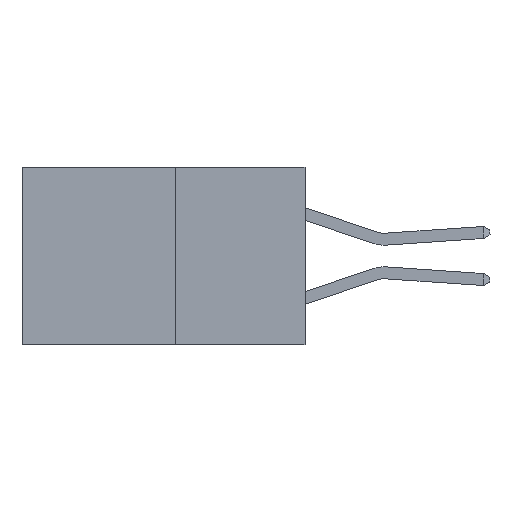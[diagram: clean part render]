
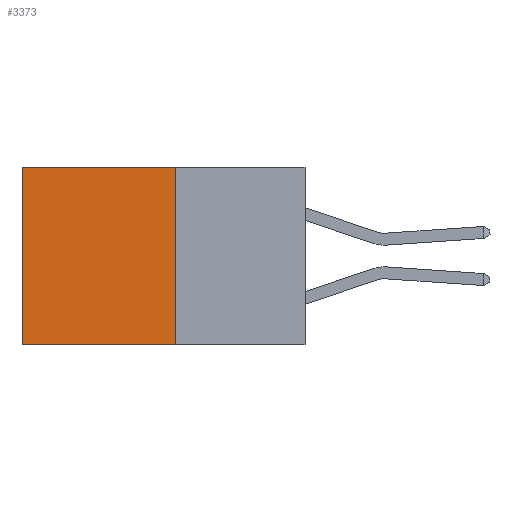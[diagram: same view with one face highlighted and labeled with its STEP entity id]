
A CAD part, left-side view. The second image highlights one B-rep face of the part: STEP entity #3373.
In plain terms, the highlighted planar face has unit normal (-1, 0, 0).
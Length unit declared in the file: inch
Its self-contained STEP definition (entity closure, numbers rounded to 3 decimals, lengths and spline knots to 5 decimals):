
#1006 = CARTESIAN_POINT ( 'NONE',  ( 0.277, 0.59, 0. ) ) ;
#1196 = CARTESIAN_POINT ( 'NONE',  ( 0.277, 0.59, -0.37 ) ) ;
#2327 = EDGE_CURVE ( 'NONE', #13616, #3309, #2424, .T. ) ;
#2424 = LINE ( 'NONE', #1196, #14204 ) ;
#3309 = VERTEX_POINT ( 'NONE', #13774 ) ;
#3373 = ADVANCED_FACE ( 'NONE', ( #16665 ), #11764, .F. ) ;
#3637 = VECTOR ( 'NONE', #19021, 39.37008 ) ;
#4277 = VERTEX_POINT ( 'NONE', #5399 ) ;
#5399 = CARTESIAN_POINT ( 'NONE',  ( 0.277, 0.27, 0. ) ) ;
#8233 = DIRECTION ( 'NONE',  ( 0., 0., -1. ) ) ;
#8403 = DIRECTION ( 'NONE',  ( 0., 0., -1. ) ) ;
#9783 = VERTEX_POINT ( 'NONE', #29953 ) ;
#9850 = LINE ( 'NONE', #25954, #3637 ) ;
#11670 = DIRECTION ( 'NONE',  ( 0., 0., -1. ) ) ;
#11732 = DIRECTION ( 'NONE',  ( 1., 0., 0. ) ) ;
#11738 = CARTESIAN_POINT ( 'NONE',  ( 0.277, 0.27, -0.37 ) ) ;
#11764 = PLANE ( 'NONE',  #20028 ) ;
#12807 = ORIENTED_EDGE ( 'NONE', *, *, #19440, .T. ) ;
#13616 = VERTEX_POINT ( 'NONE', #1006 ) ;
#13774 = CARTESIAN_POINT ( 'NONE',  ( 0.277, 0.59, -0.37 ) ) ;
#14204 = VECTOR ( 'NONE', #8233, 39.37008 ) ;
#16665 = FACE_OUTER_BOUND ( 'NONE', #19977, .T. ) ;
#16910 = EDGE_CURVE ( 'NONE', #4277, #9783, #22843, .T. ) ;
#17259 = DIRECTION ( 'NONE',  ( 0., 1., 0. ) ) ;
#17844 = ORIENTED_EDGE ( 'NONE', *, *, #25659, .F. ) ;
#19021 = DIRECTION ( 'NONE',  ( 0., 1., 0. ) ) ;
#19440 = EDGE_CURVE ( 'NONE', #4277, #13616, #9850, .T. ) ;
#19977 = EDGE_LOOP ( 'NONE', ( #21830, #17844, #25178, #12807 ) ) ;
#20028 = AXIS2_PLACEMENT_3D ( 'NONE', #11738, #11732, #11670 ) ;
#21830 = ORIENTED_EDGE ( 'NONE', *, *, #2327, .T. ) ;
#22437 = CARTESIAN_POINT ( 'NONE',  ( 0.277, 0.27, -0.37 ) ) ;
#22843 = LINE ( 'NONE', #22437, #28992 ) ;
#22852 = VECTOR ( 'NONE', #17259, 39.37008 ) ;
#25178 = ORIENTED_EDGE ( 'NONE', *, *, #16910, .F. ) ;
#25659 = EDGE_CURVE ( 'NONE', #9783, #3309, #29002, .T. ) ;
#25954 = CARTESIAN_POINT ( 'NONE',  ( 0.277, 0.27, 0. ) ) ;
#28848 = CARTESIAN_POINT ( 'NONE',  ( 0.277, 0.27, -0.37 ) ) ;
#28992 = VECTOR ( 'NONE', #8403, 39.37008 ) ;
#29002 = LINE ( 'NONE', #28848, #22852 ) ;
#29953 = CARTESIAN_POINT ( 'NONE',  ( 0.277, 0.27, -0.37 ) ) ;
